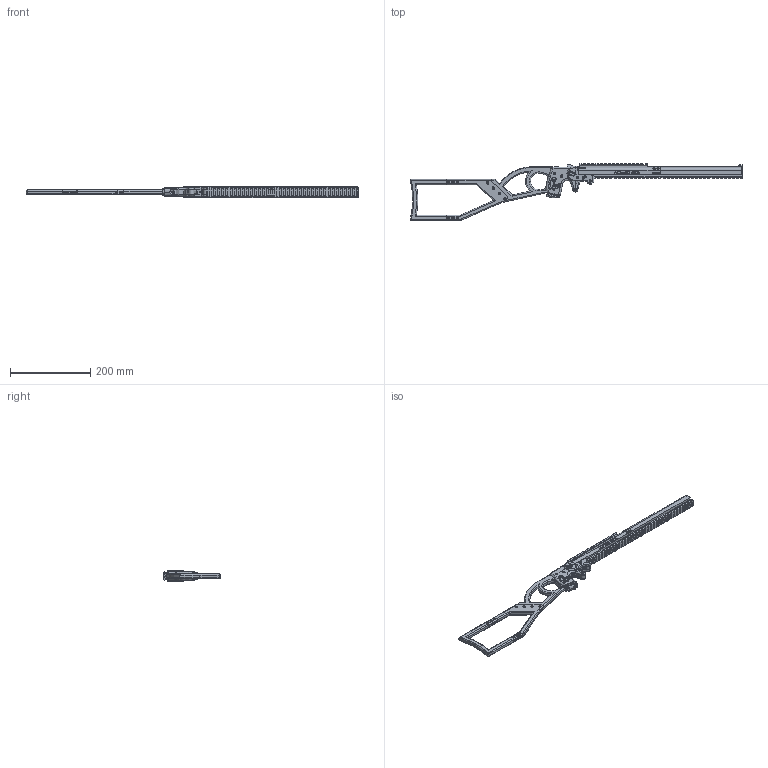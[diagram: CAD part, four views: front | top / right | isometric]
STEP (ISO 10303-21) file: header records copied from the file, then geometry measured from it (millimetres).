
FILE_DESCRIPTION (( 'STEP AP214' ), '1' );
FILE_NAME ('The Long Boi.STEP', '2022-10-19T18:53:01', ( '' ), ( '' ), 'SwSTEP 2.0', 'SolidWorks 2013', '' );
FILE_SCHEMA (( 'AUTOMOTIVE_DESIGN' ));
Length unit declared in the file: inch
Products named in the file (14): Ejector Rod; Latch; Breech Block; The Long Boi; Trigger; Stock V2 Rear_Stock; Left Side Frame; Long Boi Barrel Front; Long Boi Barrel Rear; Stock V2 Front_Stock; Right Side Frame; Ammo Storage Clip; Grip Spacer V2_Stock; Hammer
Assembly tree (13 placements, depth 2):
  The Long Boi
    Left Side Frame
    Ammo Storage Clip
    Ejector Rod
    Breech Block
    Hammer
    Latch
    Trigger
    Right Side Frame
    Long Boi Barrel Rear
    Long Boi Barrel Front
    Grip Spacer V2_Stock
    Stock V2 Front_Stock
    Stock V2 Rear_Stock
Bounding box: 825.92 x 140.95 x 27.97 mm (x, y, z)
Volume: 483688.3 mm3; surface area: 167454.1 mm2
Topology: 13 solids, 13 shells, 7429 faces, 16855 edges, 9533 vertices
Faces by surface type: plane 6762, cylinder 387, bspline 170, cone 84, torus 22, sphere 4
Entity records: 216105 total; most frequent: CARTESIAN_POINT 43664, ORIENTED_EDGE 33678, DIRECTION 31671, EDGE_CURVE 16839, LINE 15395, VECTOR 15395, VERTEX_POINT 9529, AXIS2_PLACEMENT_3D 8138
